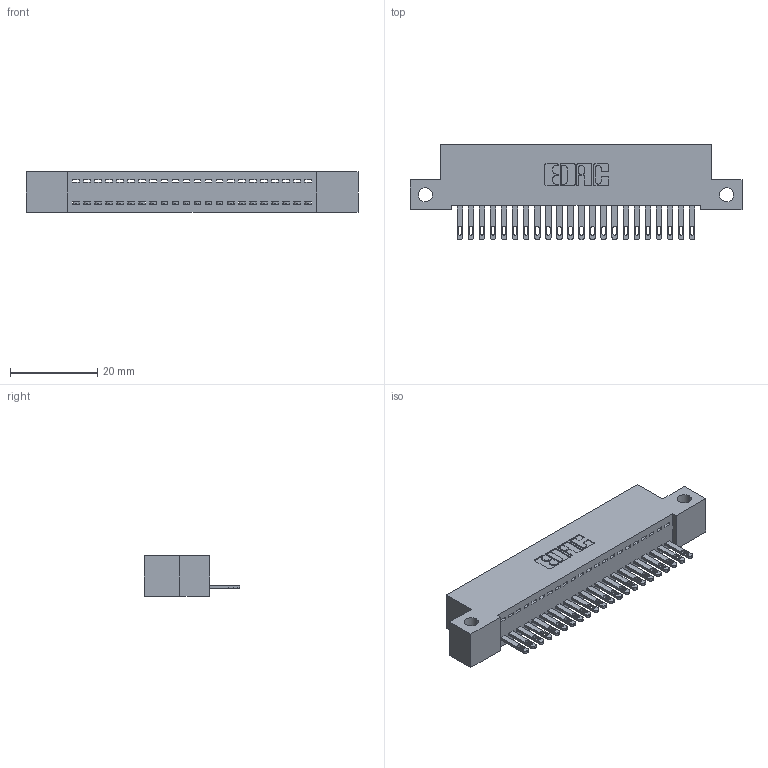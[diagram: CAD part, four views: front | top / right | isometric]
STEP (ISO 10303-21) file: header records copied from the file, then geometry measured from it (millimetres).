
FILE_DESCRIPTION (( 'STEP AP203' ), '1' );
FILE_NAME ('342-022-500-112.STEP', '2018-08-11T00:06:15', ( '' ), ( '' ), 'SwSTEP 2.0', 'SolidWorks 2016', '' );
FILE_SCHEMA (( 'CONFIG_CONTROL_DESIGN' ));
Length unit declared in the file: inch
Products named in the file (3): 342 Part_Side Mount; 345-292-001_345-293-100; 342-022-500-112
Assembly tree (23 placements, depth 2):
  342-022-500-112
    342 Part_Side Mount
    345-292-001_345-293-100  x22
Bounding box: 76.2 x 21.85 x 9.4 mm (x, y, z)
Volume: 6547.2 mm3; surface area: 9121.1 mm2
Topology: 23 solids, 23 shells, 1298 faces, 3995 edges, 2662 vertices
Faces by surface type: plane 858, cylinder 440
Entity records: 15837 total; most frequent: CARTESIAN_POINT 2740, ORIENTED_EDGE 2698, DIRECTION 2353, EDGE_CURVE 1349, LINE 1217, VECTOR 1217, VERTEX_POINT 898, AXIS2_PLACEMENT_3D 568
